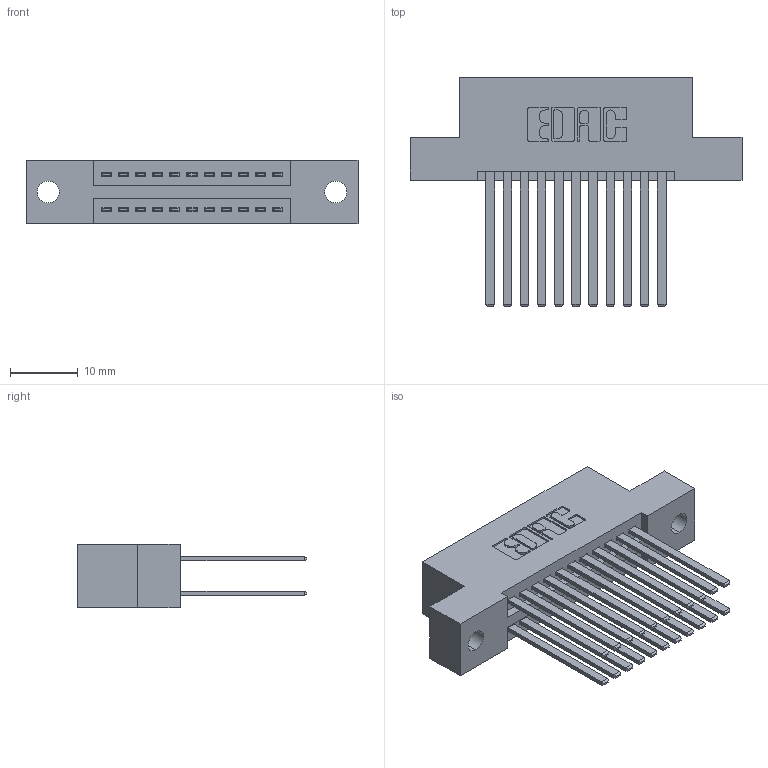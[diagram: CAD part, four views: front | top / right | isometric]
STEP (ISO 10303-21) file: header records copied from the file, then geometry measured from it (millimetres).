
FILE_DESCRIPTION (( 'STEP AP203' ), '1' );
FILE_NAME ('395-022-544-202.STEP', '2019-10-15T23:20:02', ( '' ), ( '' ), 'SwSTEP 2.0', 'SolidWorks 2016', '' );
FILE_SCHEMA (( 'CONFIG_CONTROL_DESIGN' ));
Length unit declared in the file: inch
Products named in the file (3): 345 Part_Flush Mounting Lugs - 0.128 Dia; 345-292-001_345-293-144; 395-022-544-202
Assembly tree (23 placements, depth 2):
  395-022-544-202
    345 Part_Flush Mounting Lugs - 0.128 Dia
    345-292-001_345-293-144  x22
Bounding box: 49.15 x 33.96 x 9.4 mm (x, y, z)
Volume: 4758.3 mm3; surface area: 7064.4 mm2
Topology: 23 solids, 23 shells, 1094 faces, 3223 edges, 2118 vertices
Faces by surface type: plane 718, cylinder 376
Entity records: 12623 total; most frequent: CARTESIAN_POINT 2144, ORIENTED_EDGE 2078, DIRECTION 1927, EDGE_CURVE 1039, LINE 867, VECTOR 867, VERTEX_POINT 690, AXIS2_PLACEMENT_3D 530
